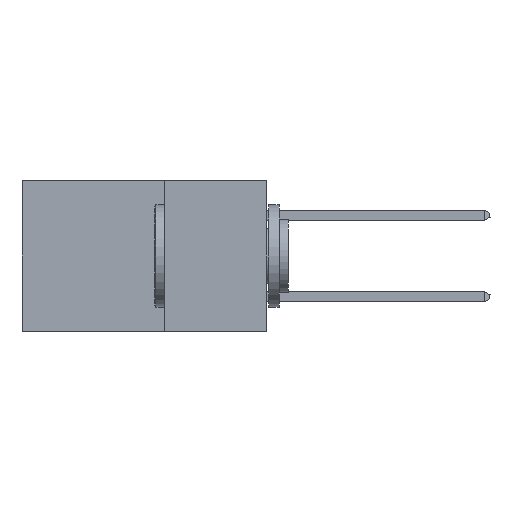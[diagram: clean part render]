
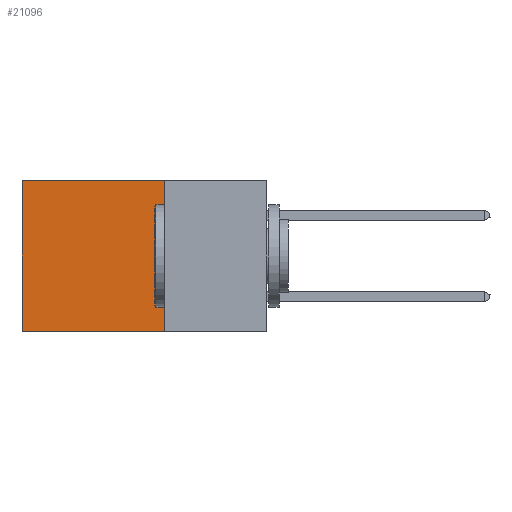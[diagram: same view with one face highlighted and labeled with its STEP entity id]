
A CAD part, left-side view. The second image highlights one B-rep face of the part: STEP entity #21096.
In plain terms, the highlighted planar face has unit normal (-1, 0, 0).
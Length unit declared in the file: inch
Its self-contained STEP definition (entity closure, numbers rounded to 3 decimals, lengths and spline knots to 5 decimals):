
#434 = AXIS2_PLACEMENT_3D ( 'NONE', #12457, #4121, #1229 ) ;
#1229 = DIRECTION ( 'NONE',  ( 0., 0., -1. ) ) ;
#2147 = LINE ( 'NONE', #13119, #35880 ) ;
#3924 = LINE ( 'NONE', #16462, #30216 ) ;
#4121 = DIRECTION ( 'NONE',  ( 1., 0., 0. ) ) ;
#5802 = LINE ( 'NONE', #13264, #27726 ) ;
#5966 = CARTESIAN_POINT ( 'NONE',  ( 0.2875, 0.25, 0. ) ) ;
#6265 = EDGE_LOOP ( 'NONE', ( #31527, #35018, #21238, #13076 ) ) ;
#6976 = LINE ( 'NONE', #35439, #27113 ) ;
#6979 = EDGE_CURVE ( 'NONE', #32496, #28390, #3924, .T. ) ;
#12457 = CARTESIAN_POINT ( 'NONE',  ( 0.2875, 0.25, 0. ) ) ;
#12874 = DIRECTION ( 'NONE',  ( 0., 0., -1. ) ) ;
#13020 = DIRECTION ( 'NONE',  ( 0., 0., -1. ) ) ;
#13076 = ORIENTED_EDGE ( 'NONE', *, *, #6979, .T. ) ;
#13119 = CARTESIAN_POINT ( 'NONE',  ( 0.2875, 0.6, 0. ) ) ;
#13264 = CARTESIAN_POINT ( 'NONE',  ( 0.2875, 0.25, -0.37 ) ) ;
#14928 = EDGE_CURVE ( 'NONE', #32496, #15079, #6976, .T. ) ;
#15079 = VERTEX_POINT ( 'NONE', #27893 ) ;
#16462 = CARTESIAN_POINT ( 'NONE',  ( 0.2875, 0.25, 0. ) ) ;
#21096 = ADVANCED_FACE ( 'NONE', ( #24279 ), #32207, .F. ) ;
#21238 = ORIENTED_EDGE ( 'NONE', *, *, #14928, .F. ) ;
#21788 = CARTESIAN_POINT ( 'NONE',  ( 0.2875, 0.6, -0.37 ) ) ;
#23674 = EDGE_CURVE ( 'NONE', #28390, #25478, #2147, .T. ) ;
#24279 = FACE_OUTER_BOUND ( 'NONE', #6265, .T. ) ;
#24896 = EDGE_CURVE ( 'NONE', #15079, #25478, #5802, .T. ) ;
#25478 = VERTEX_POINT ( 'NONE', #21788 ) ;
#27113 = VECTOR ( 'NONE', #13020, 39.37008 ) ;
#27726 = VECTOR ( 'NONE', #29928, 39.37008 ) ;
#27893 = CARTESIAN_POINT ( 'NONE',  ( 0.2875, 0.25, -0.37 ) ) ;
#28390 = VERTEX_POINT ( 'NONE', #35184 ) ;
#29928 = DIRECTION ( 'NONE',  ( 0., 1., 0. ) ) ;
#30216 = VECTOR ( 'NONE', #35736, 39.37008 ) ;
#31527 = ORIENTED_EDGE ( 'NONE', *, *, #23674, .T. ) ;
#32207 = PLANE ( 'NONE',  #434 ) ;
#32496 = VERTEX_POINT ( 'NONE', #5966 ) ;
#35018 = ORIENTED_EDGE ( 'NONE', *, *, #24896, .F. ) ;
#35184 = CARTESIAN_POINT ( 'NONE',  ( 0.2875, 0.6, 0. ) ) ;
#35439 = CARTESIAN_POINT ( 'NONE',  ( 0.2875, 0.25, 0. ) ) ;
#35736 = DIRECTION ( 'NONE',  ( 0., 1., 0. ) ) ;
#35880 = VECTOR ( 'NONE', #12874, 39.37008 ) ;
